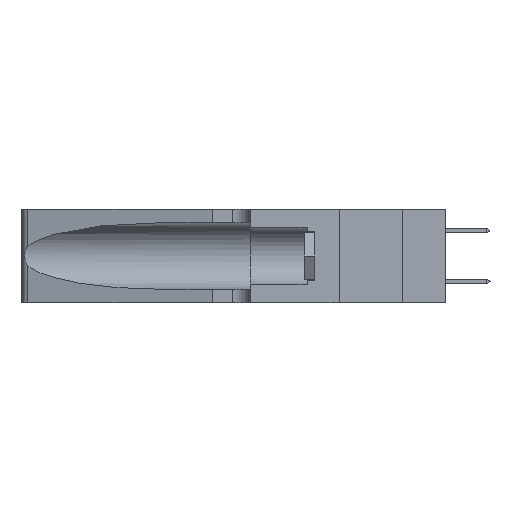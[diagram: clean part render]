
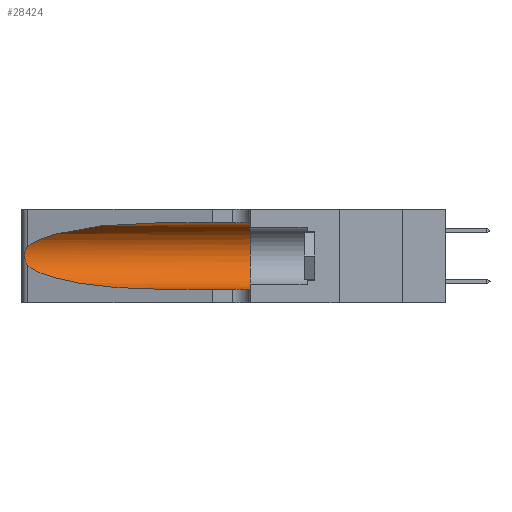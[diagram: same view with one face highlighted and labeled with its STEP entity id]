
A CAD part, left-side view. The second image highlights one B-rep face of the part: STEP entity #28424.
In plain terms, the highlighted cylindrical face has radius 3.308 mm (diameter 6.617 mm), a partial arc.
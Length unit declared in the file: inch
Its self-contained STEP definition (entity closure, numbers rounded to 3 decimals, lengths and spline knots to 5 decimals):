
#126 = CARTESIAN_POINT ( 'NONE',  ( 0.25854, 1.2359, 0.20912 ) ) ;
#1006 = AXIS2_PLACEMENT_3D ( 'NONE', #1634, #16017, #6857 ) ;
#1195 = CARTESIAN_POINT ( 'NONE',  ( 0.25639, 1.23186, 0.15144 ) ) ;
#1551 = EDGE_CURVE ( 'NONE', #15769, #10796, #1838, .T. ) ;
#1634 = CARTESIAN_POINT ( 'NONE',  ( 0.1305, 1.61858, 0.185 ) ) ;
#1835 = CARTESIAN_POINT ( 'NONE',  ( 0.1305, 0.72297, 0.31525 ) ) ;
#1838 =( BOUNDED_CURVE ( )  B_SPLINE_CURVE ( 3, ( #32260, #15737, #20943, #20737 ),
 .UNSPECIFIED., .F., .T. ) 
 B_SPLINE_CURVE_WITH_KNOTS ( ( 4, 4 ),
 ( 3.44316, 4.71239 ),
 .UNSPECIFIED. ) 
 CURVE ( )  GEOMETRIC_REPRESENTATION_ITEM ( )  RATIONAL_B_SPLINE_CURVE ( ( 1., 0.87, 0.87, 1. ) ) 
 REPRESENTATION_ITEM ( '' )  );
#2590 = EDGE_CURVE ( 'NONE', #27474, #17490, #24974, .T. ) ;
#2930 = CARTESIAN_POINT ( 'NONE',  ( 0.1305, 1.61858, 0.05475 ) ) ;
#3445 = CARTESIAN_POINT ( 'NONE',  ( 0.25555, 1.22993, 0.14849 ) ) ;
#3564 = CARTESIAN_POINT ( 'NONE',  ( 0.25856, 1.23593, 0.16098 ) ) ;
#3908 = VERTEX_POINT ( 'NONE', #6978 ) ;
#4458 = CARTESIAN_POINT ( 'NONE',  ( 0.25487, 1.22718, 0.22369 ) ) ;
#5975 = CARTESIAN_POINT ( 'NONE',  ( 0.25789, 1.23486, 0.15765 ) ) ;
#6184 = ORIENTED_EDGE ( 'NONE', *, *, #2590, .T. ) ;
#6310 = B_SPLINE_CURVE_WITH_KNOTS ( 'NONE', 3,
 ( #4458, #27004, #12418, #25348, #126, #26101, #13819, #31114, #18917, #3564, #5975, #1195, #3445, #21142 ),
 .UNSPECIFIED., .F., .F.,
 ( 4, 2, 2, 2, 2, 2, 4 ),
 ( 0., 0.00027, 0.00053, 0.00107, 0.0016, 0.00187, 0.00214 ),
 .UNSPECIFIED. ) ;
#6857 = DIRECTION ( 'NONE',  ( 0., 0., -1. ) ) ;
#6978 = CARTESIAN_POINT ( 'NONE',  ( 0.1305, 0.35, 0.05475 ) ) ;
#7106 = DIRECTION ( 'NONE',  ( 0., 1., 0. ) ) ;
#7388 = CARTESIAN_POINT ( 'NONE',  ( 0.1305, 1.61858, 0.31525 ) ) ;
#7405 = ORIENTED_EDGE ( 'NONE', *, *, #13243, .F. ) ;
#7581 = VERTEX_POINT ( 'NONE', #23480 ) ;
#8734 = VECTOR ( 'NONE', #22312, 39.37008 ) ;
#9517 = LINE ( 'NONE', #7388, #8734 ) ;
#9543 = DIRECTION ( 'NONE',  ( 0., 0., 1. ) ) ;
#10796 = VERTEX_POINT ( 'NONE', #26676 ) ;
#11254 = FACE_OUTER_BOUND ( 'NONE', #21007, .T. ) ;
#11895 = CARTESIAN_POINT ( 'NONE',  ( 0.25487, 1.22718, 0.22369 ) ) ;
#12418 = CARTESIAN_POINT ( 'NONE',  ( 0.25639, 1.23184, 0.21858 ) ) ;
#13243 = EDGE_CURVE ( 'NONE', #27474, #7581, #9517, .T. ) ;
#13765 = AXIS2_PLACEMENT_3D ( 'NONE', #24589, #7106, #9543 ) ;
#13819 = CARTESIAN_POINT ( 'NONE',  ( 0.26075, 1.23896, 0.19203 ) ) ;
#15737 = CARTESIAN_POINT ( 'NONE',  ( 0.2373, 1.15595, 0.08982 ) ) ;
#15769 = VERTEX_POINT ( 'NONE', #31415 ) ;
#16017 = DIRECTION ( 'NONE',  ( 0., -1., 0. ) ) ;
#16946 = CIRCLE ( 'NONE', #13765, 0.13025 ) ;
#17431 = ORIENTED_EDGE ( 'NONE', *, *, #1551, .T. ) ;
#17490 = VERTEX_POINT ( 'NONE', #11895 ) ;
#17698 = LINE ( 'NONE', #2930, #32760 ) ;
#18073 = EDGE_CURVE ( 'NONE', #17490, #15769, #6310, .T. ) ;
#18917 = CARTESIAN_POINT ( 'NONE',  ( 0.26017, 1.23833, 0.17102 ) ) ;
#20542 = ORIENTED_EDGE ( 'NONE', *, *, #18073, .T. ) ;
#20737 = CARTESIAN_POINT ( 'NONE',  ( 0.1305, 0.72297, 0.05475 ) ) ;
#20943 = CARTESIAN_POINT ( 'NONE',  ( 0.18966, 0.96281, 0.05475 ) ) ;
#21007 = EDGE_LOOP ( 'NONE', ( #6184, #20542, #17431, #24663, #29918, #7405 ) ) ;
#21142 = CARTESIAN_POINT ( 'NONE',  ( 0.25487, 1.22718, 0.14631 ) ) ;
#21746 = CARTESIAN_POINT ( 'NONE',  ( 0.25487, 1.22718, 0.22369 ) ) ;
#22312 = DIRECTION ( 'NONE',  ( 0., -1., 0. ) ) ;
#22559 = EDGE_CURVE ( 'NONE', #10796, #3908, #17698, .T. ) ;
#22820 = EDGE_CURVE ( 'NONE', #7581, #3908, #16946, .T. ) ;
#23480 = CARTESIAN_POINT ( 'NONE',  ( 0.1305, 0.35, 0.31525 ) ) ;
#24589 = CARTESIAN_POINT ( 'NONE',  ( 0.1305, 0.35, 0.185 ) ) ;
#24663 = ORIENTED_EDGE ( 'NONE', *, *, #22559, .T. ) ;
#24974 =( BOUNDED_CURVE ( )  B_SPLINE_CURVE ( 3, ( #1835, #31955, #26820, #21746 ),
 .UNSPECIFIED., .F., .F. ) 
 B_SPLINE_CURVE_WITH_KNOTS ( ( 4, 4 ),
 ( 1.5708, 2.84003 ),
 .UNSPECIFIED. ) 
 CURVE ( )  GEOMETRIC_REPRESENTATION_ITEM ( )  RATIONAL_B_SPLINE_CURVE ( ( 1., 0.87, 0.87, 1. ) ) 
 REPRESENTATION_ITEM ( '' )  );
#25348 = CARTESIAN_POINT ( 'NONE',  ( 0.25787, 1.23484, 0.2124 ) ) ;
#26101 = CARTESIAN_POINT ( 'NONE',  ( 0.26018, 1.23835, 0.19895 ) ) ;
#26676 = CARTESIAN_POINT ( 'NONE',  ( 0.1305, 0.72297, 0.05475 ) ) ;
#26820 = CARTESIAN_POINT ( 'NONE',  ( 0.2373, 1.15595, 0.28018 ) ) ;
#27004 = CARTESIAN_POINT ( 'NONE',  ( 0.25555, 1.22994, 0.2215 ) ) ;
#27474 = VERTEX_POINT ( 'NONE', #27571 ) ;
#27571 = CARTESIAN_POINT ( 'NONE',  ( 0.1305, 0.72297, 0.31525 ) ) ;
#28424 = ADVANCED_FACE ( 'NONE', ( #11254 ), #31839, .F. ) ;
#29918 = ORIENTED_EDGE ( 'NONE', *, *, #22820, .F. ) ;
#30917 = DIRECTION ( 'NONE',  ( 0., -1., 0. ) ) ;
#31114 = CARTESIAN_POINT ( 'NONE',  ( 0.26075, 1.23896, 0.178 ) ) ;
#31415 = CARTESIAN_POINT ( 'NONE',  ( 0.25487, 1.22718, 0.14631 ) ) ;
#31839 = CYLINDRICAL_SURFACE ( 'NONE', #1006, 0.13025 ) ;
#31955 = CARTESIAN_POINT ( 'NONE',  ( 0.18966, 0.96281, 0.31525 ) ) ;
#32260 = CARTESIAN_POINT ( 'NONE',  ( 0.25487, 1.22718, 0.14631 ) ) ;
#32760 = VECTOR ( 'NONE', #30917, 39.37008 ) ;
